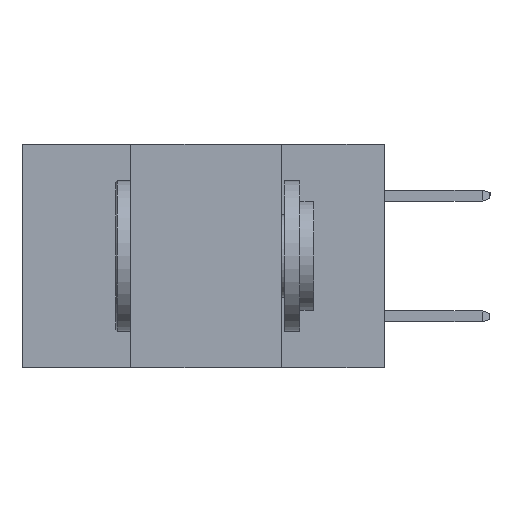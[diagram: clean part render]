
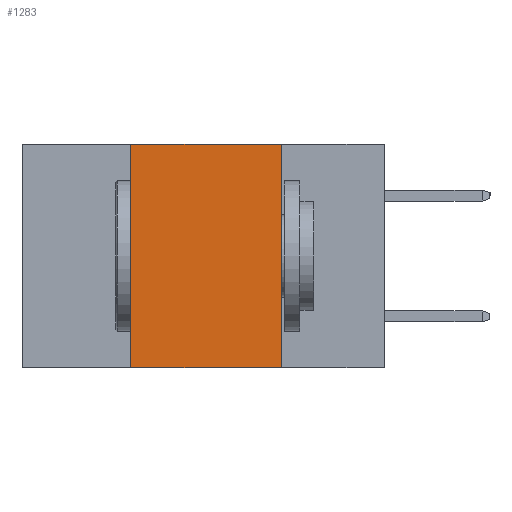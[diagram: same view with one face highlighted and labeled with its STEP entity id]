
A CAD part, left-side view. The second image highlights one B-rep face of the part: STEP entity #1283.
In plain terms, the highlighted planar face has unit normal (-1, 0, 0).
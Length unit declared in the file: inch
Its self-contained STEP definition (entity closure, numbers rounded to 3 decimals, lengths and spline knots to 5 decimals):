
#976 = DIRECTION ( 'NONE',  ( 1., 0., 0. ) ) ;
#1283 = ADVANCED_FACE ( 'NONE', ( #4961 ), #1877, .F. ) ;
#1818 = LINE ( 'NONE', #9228, #3420 ) ;
#1844 = LINE ( 'NONE', #3563, #2140 ) ;
#1877 = PLANE ( 'NONE',  #5503 ) ;
#2045 = EDGE_CURVE ( 'NONE', #3392, #3321, #10393, .T. ) ;
#2057 = VERTEX_POINT ( 'NONE', #3157 ) ;
#2140 = VECTOR ( 'NONE', #5084, 39.37008 ) ;
#2611 = DIRECTION ( 'NONE',  ( 0., 0., -1. ) ) ;
#3114 = CARTESIAN_POINT ( 'NONE',  ( 0., 0.17, 0. ) ) ;
#3157 = CARTESIAN_POINT ( 'NONE',  ( 0., 0.42, -0.37 ) ) ;
#3321 = VERTEX_POINT ( 'NONE', #3114 ) ;
#3392 = VERTEX_POINT ( 'NONE', #7216 ) ;
#3420 = VECTOR ( 'NONE', #8282, 39.37008 ) ;
#3563 = CARTESIAN_POINT ( 'NONE',  ( 0., 0.42, -0.37 ) ) ;
#3733 = VERTEX_POINT ( 'NONE', #7091 ) ;
#3940 = ORIENTED_EDGE ( 'NONE', *, *, #2045, .F. ) ;
#3989 = EDGE_LOOP ( 'NONE', ( #4611, #3940, #4790, #8812 ) ) ;
#4276 = EDGE_CURVE ( 'NONE', #3321, #3733, #4352, .T. ) ;
#4303 = EDGE_CURVE ( 'NONE', #2057, #3733, #1818, .T. ) ;
#4352 = LINE ( 'NONE', #5915, #8691 ) ;
#4611 = ORIENTED_EDGE ( 'NONE', *, *, #4276, .F. ) ;
#4790 = ORIENTED_EDGE ( 'NONE', *, *, #8092, .F. ) ;
#4961 = FACE_OUTER_BOUND ( 'NONE', #3989, .T. ) ;
#5084 = DIRECTION ( 'NONE',  ( 0., 0., 1. ) ) ;
#5114 = VECTOR ( 'NONE', #6520, 39.37008 ) ;
#5503 = AXIS2_PLACEMENT_3D ( 'NONE', #5769, #976, #2611 ) ;
#5769 = CARTESIAN_POINT ( 'NONE',  ( 0., 0.6, 0. ) ) ;
#5915 = CARTESIAN_POINT ( 'NONE',  ( 0., 0.17, -0.37 ) ) ;
#6520 = DIRECTION ( 'NONE',  ( 0., -1., 0. ) ) ;
#7091 = CARTESIAN_POINT ( 'NONE',  ( 0., 0.17, -0.37 ) ) ;
#7216 = CARTESIAN_POINT ( 'NONE',  ( 0., 0.42, 0. ) ) ;
#7990 = CARTESIAN_POINT ( 'NONE',  ( 0., 0.6, 0. ) ) ;
#8092 = EDGE_CURVE ( 'NONE', #2057, #3392, #1844, .T. ) ;
#8282 = DIRECTION ( 'NONE',  ( 0., -1., 0. ) ) ;
#8691 = VECTOR ( 'NONE', #9795, 39.37008 ) ;
#8812 = ORIENTED_EDGE ( 'NONE', *, *, #4303, .T. ) ;
#9228 = CARTESIAN_POINT ( 'NONE',  ( 0., 0.6, -0.37 ) ) ;
#9795 = DIRECTION ( 'NONE',  ( 0., 0., -1. ) ) ;
#10393 = LINE ( 'NONE', #7990, #5114 ) ;
